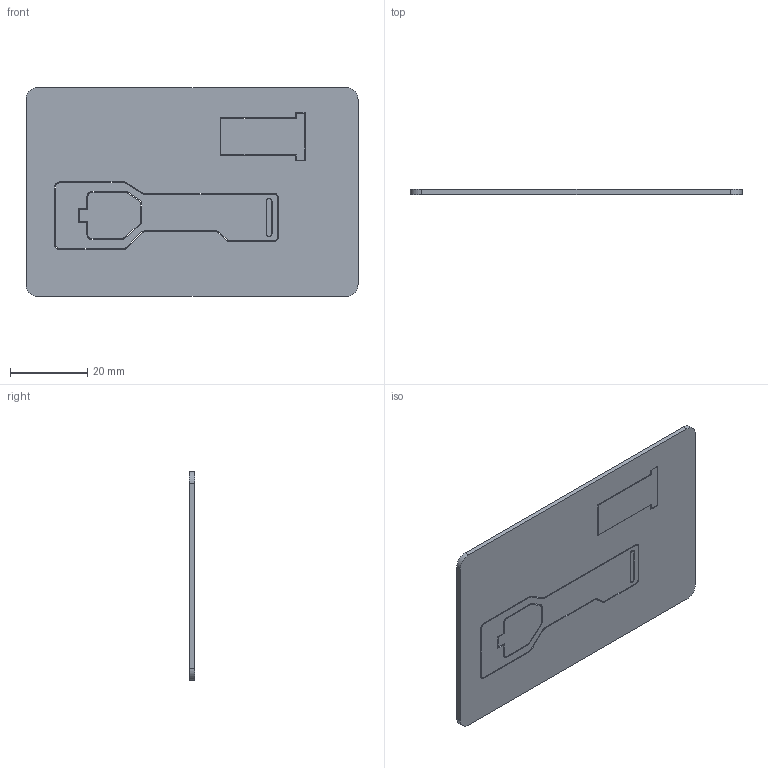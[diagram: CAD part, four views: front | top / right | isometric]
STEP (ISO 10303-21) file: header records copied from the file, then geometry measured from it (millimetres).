
FILE_DESCRIPTION (( 'STEP AP214' ), '1' );
FILE_NAME ('card.STEP', '2021-03-08T22:39:28', ( '' ), ( '' ), 'SwSTEP 2.0', 'SolidWorks 2019', '' );
FILE_SCHEMA (( 'AUTOMOTIVE_DESIGN' ));
Length unit declared in the file: millimetre
Products named in the file (1): card
Bounding box: 86 x 1.3 x 54 mm (x, y, z)
Volume: 5945.5 mm3; surface area: 10250.8 mm2
Topology: 5 solids, 5 shells, 116 faces, 318 edges, 212 vertices
Faces by surface type: plane 74, cylinder 42
Entity records: 3772 total; most frequent: CARTESIAN_POINT 647, DIRECTION 636, ORIENTED_EDGE 636, EDGE_CURVE 318, LINE 234, VECTOR 234, VERTEX_POINT 212, AXIS2_PLACEMENT_3D 201
